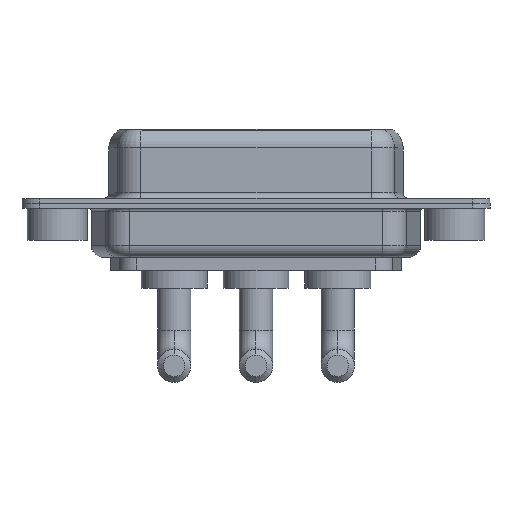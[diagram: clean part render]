
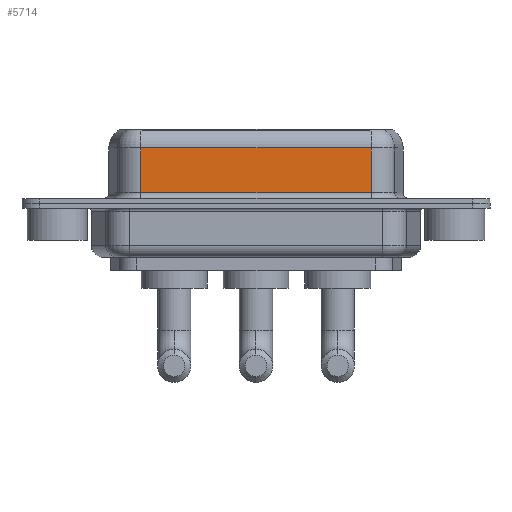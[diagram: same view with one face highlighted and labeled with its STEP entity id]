
A CAD part, front view. The second image highlights one B-rep face of the part: STEP entity #5714.
In plain terms, the highlighted planar face has unit normal (0, -1, 0).
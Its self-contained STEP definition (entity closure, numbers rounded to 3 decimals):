
#106 = EDGE_CURVE ( 'NONE', #409, #856, #7273, .T. ) ;
#409 = VERTEX_POINT ( 'NONE', #2981 ) ;
#856 = VERTEX_POINT ( 'NONE', #10539 ) ;
#1067 = DIRECTION ( 'NONE',  ( -1., 0., 0. ) ) ;
#1517 = CARTESIAN_POINT ( 'NONE',  ( 26.287, -3.95, 6.4 ) ) ;
#1750 = DIRECTION ( 'NONE',  ( 0., 0., -1. ) ) ;
#1839 = DIRECTION ( 'NONE',  ( 0., 0., 1. ) ) ;
#1936 = LINE ( 'NONE', #9624, #8286 ) ;
#2066 = VERTEX_POINT ( 'NONE', #9163 ) ;
#2312 = VECTOR ( 'NONE', #1750, 1000. ) ;
#2336 = EDGE_CURVE ( 'NONE', #2066, #856, #8772, .T. ) ;
#2342 = ORIENTED_EDGE ( 'NONE', *, *, #2336, .T. ) ;
#2981 = CARTESIAN_POINT ( 'NONE',  ( 26.287, -3.95, 4.65 ) ) ;
#3772 = EDGE_CURVE ( 'NONE', #409, #11224, #1936, .T. ) ;
#4010 = CARTESIAN_POINT ( 'NONE',  ( 26.287, -3.95, 0.9 ) ) ;
#4049 = ORIENTED_EDGE ( 'NONE', *, *, #7770, .T. ) ;
#4127 = LINE ( 'NONE', #11737, #5620 ) ;
#5137 = ORIENTED_EDGE ( 'NONE', *, *, #106, .F. ) ;
#5252 = AXIS2_PLACEMENT_3D ( 'NONE', #11390, #10628, #1839 ) ;
#5620 = VECTOR ( 'NONE', #6814, 1000. ) ;
#5714 = ADVANCED_FACE ( 'NONE', ( #9529 ), #11558, .F. ) ;
#5837 = CARTESIAN_POINT ( 'NONE',  ( 7.013, -3.95, 4.65 ) ) ;
#6814 = DIRECTION ( 'NONE',  ( 0., 0., -1. ) ) ;
#7273 = LINE ( 'NONE', #1517, #2312 ) ;
#7611 = VECTOR ( 'NONE', #8833, 1000. ) ;
#7770 = EDGE_CURVE ( 'NONE', #11224, #2066, #4127, .T. ) ;
#8286 = VECTOR ( 'NONE', #1067, 1000. ) ;
#8676 = ORIENTED_EDGE ( 'NONE', *, *, #3772, .T. ) ;
#8772 = LINE ( 'NONE', #4010, #7611 ) ;
#8833 = DIRECTION ( 'NONE',  ( 1., 0., 0. ) ) ;
#9163 = CARTESIAN_POINT ( 'NONE',  ( 7.013, -3.95, 0.9 ) ) ;
#9529 = FACE_OUTER_BOUND ( 'NONE', #11949, .T. ) ;
#9624 = CARTESIAN_POINT ( 'NONE',  ( 26.287, -3.95, 4.65 ) ) ;
#10539 = CARTESIAN_POINT ( 'NONE',  ( 26.287, -3.95, 0.9 ) ) ;
#10628 = DIRECTION ( 'NONE',  ( 0., 1., 0. ) ) ;
#11224 = VERTEX_POINT ( 'NONE', #5837 ) ;
#11390 = CARTESIAN_POINT ( 'NONE',  ( 26.287, -3.95, 6.4 ) ) ;
#11558 = PLANE ( 'NONE',  #5252 ) ;
#11737 = CARTESIAN_POINT ( 'NONE',  ( 7.013, -3.95, 6.4 ) ) ;
#11949 = EDGE_LOOP ( 'NONE', ( #5137, #8676, #4049, #2342 ) ) ;
